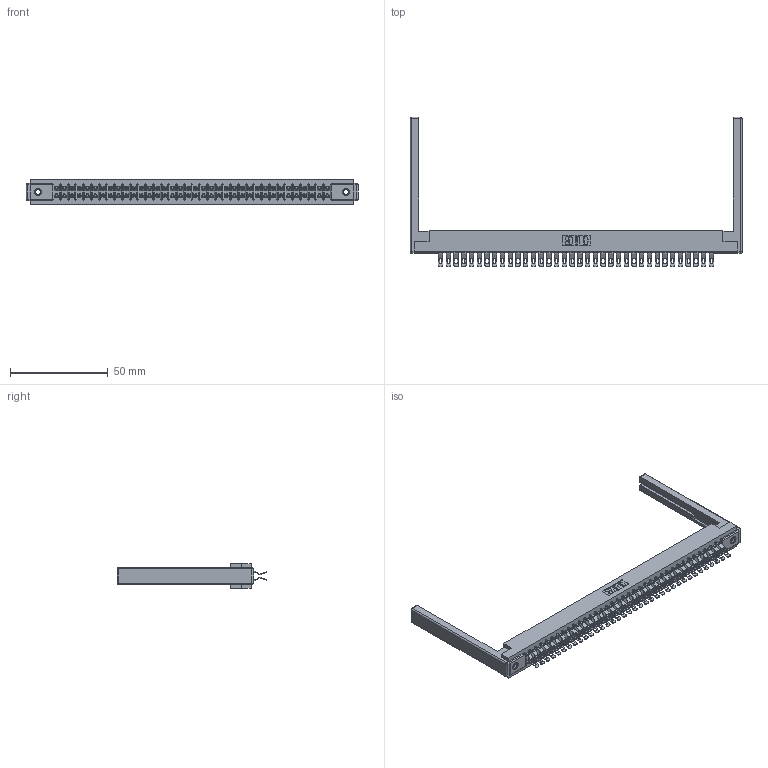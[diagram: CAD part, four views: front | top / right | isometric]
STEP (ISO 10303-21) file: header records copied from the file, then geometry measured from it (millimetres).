
FILE_DESCRIPTION (( 'STEP AP203' ), '1' );
FILE_NAME ('307-072-555-268.STEP', '2019-09-06T20:31:13', ( '' ), ( '' ), 'SwSTEP 2.0', 'SolidWorks 2016', '' );
FILE_SCHEMA (( 'CONFIG_CONTROL_DESIGN' ));
Length unit declared in the file: inch
Products named in the file (5): 307 Part_.156 Dia Mounting Holes; 307-290-001_555; 307-220-068; 307-072-555-268; 345-250-001_345-250-001-102
Assembly tree (77 placements, depth 2):
  307-072-555-268
    307 Part_.156 Dia Mounting Holes
    307-290-001_555  x72
    307-220-068  x2
    345-250-001_345-250-001-102  x2
Bounding box: 170.08 x 76.71 x 12.7 mm (x, y, z)
Volume: 22638.4 mm3; surface area: 27391 mm2
Topology: 77 solids, 77 shells, 4701 faces, 13745 edges, 8946 vertices
Faces by surface type: plane 2606, cylinder 1997, sphere 82, cone 12, torus 4
Entity records: 36050 total; most frequent: CARTESIAN_POINT 5881, ORIENTED_EDGE 5822, DIRECTION 5785, EDGE_CURVE 2911, VECTOR 2217, LINE 2217, VERTEX_POINT 1880, AXIS2_PLACEMENT_3D 1784
